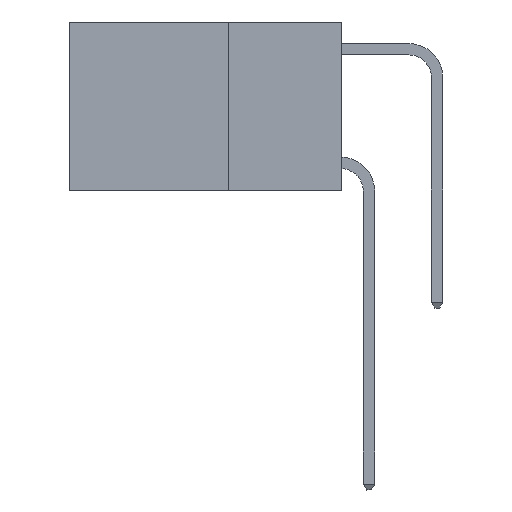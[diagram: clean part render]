
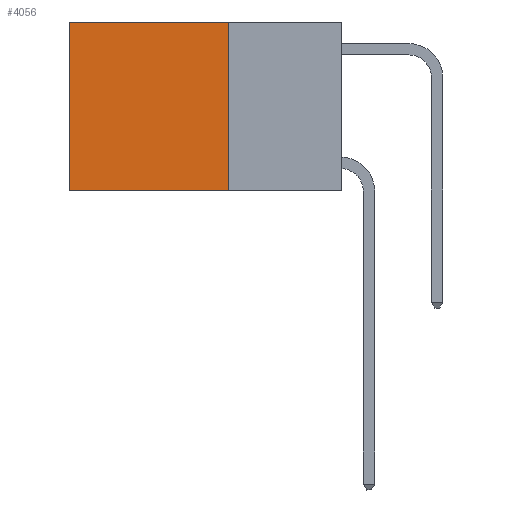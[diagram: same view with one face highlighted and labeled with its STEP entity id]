
A CAD part, left-side view. The second image highlights one B-rep face of the part: STEP entity #4056.
In plain terms, the highlighted planar face has unit normal (-1, 0, 0).
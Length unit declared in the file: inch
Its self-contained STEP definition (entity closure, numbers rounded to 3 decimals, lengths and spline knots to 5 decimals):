
#28 = ORIENTED_EDGE ( 'NONE', *, *, #12712, .F. ) ;
#735 = DIRECTION ( 'NONE',  ( 0., 0., -1. ) ) ;
#1060 = CARTESIAN_POINT ( 'NONE',  ( 0.2625, 0.25, 0. ) ) ;
#1678 = VECTOR ( 'NONE', #21158, 39.37008 ) ;
#1846 = VERTEX_POINT ( 'NONE', #12123 ) ;
#2671 = AXIS2_PLACEMENT_3D ( 'NONE', #8195, #7978, #14573 ) ;
#2747 = CARTESIAN_POINT ( 'NONE',  ( 0.2625, 0.6, -0.37 ) ) ;
#2934 = LINE ( 'NONE', #21300, #11900 ) ;
#2994 = VECTOR ( 'NONE', #18717, 39.37008 ) ;
#3715 = ORIENTED_EDGE ( 'NONE', *, *, #15023, .F. ) ;
#4056 = ADVANCED_FACE ( 'NONE', ( #9815 ), #16194, .F. ) ;
#4316 = CARTESIAN_POINT ( 'NONE',  ( 0.2625, 0.25, -0.37 ) ) ;
#4841 = VERTEX_POINT ( 'NONE', #4316 ) ;
#5862 = EDGE_LOOP ( 'NONE', ( #5869, #28, #3715, #11839 ) ) ;
#5869 = ORIENTED_EDGE ( 'NONE', *, *, #10209, .T. ) ;
#6391 = DIRECTION ( 'NONE',  ( 0., 0., -1. ) ) ;
#7978 = DIRECTION ( 'NONE',  ( 1., 0., 0. ) ) ;
#8195 = CARTESIAN_POINT ( 'NONE',  ( 0.2625, 0.25, 0. ) ) ;
#9815 = FACE_OUTER_BOUND ( 'NONE', #5862, .T. ) ;
#10209 = EDGE_CURVE ( 'NONE', #1846, #20970, #2934, .T. ) ;
#11839 = ORIENTED_EDGE ( 'NONE', *, *, #15270, .T. ) ;
#11900 = VECTOR ( 'NONE', #6391, 39.37008 ) ;
#12123 = CARTESIAN_POINT ( 'NONE',  ( 0.2625, 0.6, 0. ) ) ;
#12712 = EDGE_CURVE ( 'NONE', #4841, #20970, #13686, .T. ) ;
#13686 = LINE ( 'NONE', #20367, #2994 ) ;
#14573 = DIRECTION ( 'NONE',  ( 0., 0., -1. ) ) ;
#15023 = EDGE_CURVE ( 'NONE', #20037, #4841, #17270, .T. ) ;
#15270 = EDGE_CURVE ( 'NONE', #20037, #1846, #19539, .T. ) ;
#16194 = PLANE ( 'NONE',  #2671 ) ;
#17270 = LINE ( 'NONE', #1060, #18552 ) ;
#17796 = CARTESIAN_POINT ( 'NONE',  ( 0.2625, 0.25, 0. ) ) ;
#18552 = VECTOR ( 'NONE', #735, 39.37008 ) ;
#18578 = CARTESIAN_POINT ( 'NONE',  ( 0.2625, 0.25, 0. ) ) ;
#18717 = DIRECTION ( 'NONE',  ( 0., 1., 0. ) ) ;
#19539 = LINE ( 'NONE', #17796, #1678 ) ;
#20037 = VERTEX_POINT ( 'NONE', #18578 ) ;
#20367 = CARTESIAN_POINT ( 'NONE',  ( 0.2625, 0.25, -0.37 ) ) ;
#20970 = VERTEX_POINT ( 'NONE', #2747 ) ;
#21158 = DIRECTION ( 'NONE',  ( 0., 1., 0. ) ) ;
#21300 = CARTESIAN_POINT ( 'NONE',  ( 0.2625, 0.6, 0. ) ) ;
